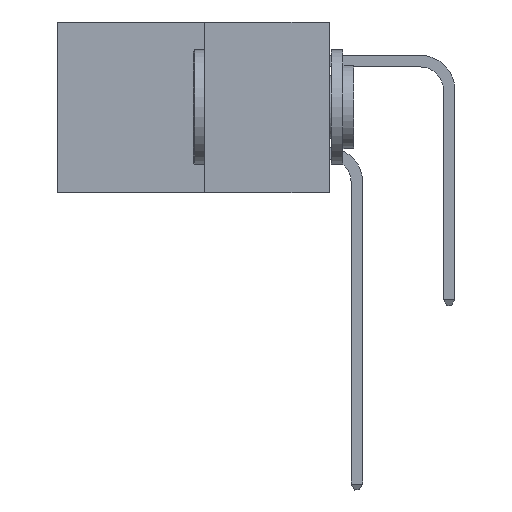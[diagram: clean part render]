
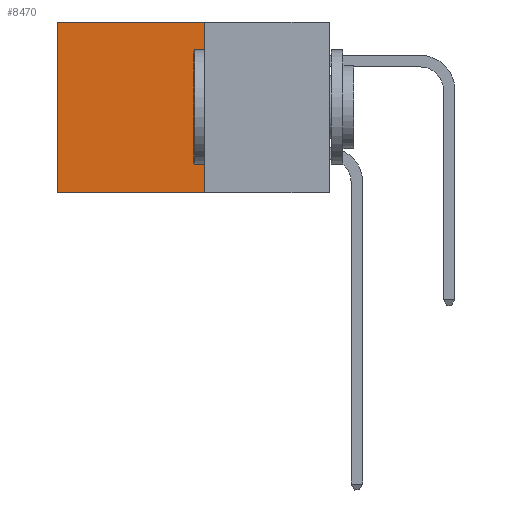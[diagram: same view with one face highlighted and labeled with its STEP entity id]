
A CAD part, left-side view. The second image highlights one B-rep face of the part: STEP entity #8470.
In plain terms, the highlighted planar face has unit normal (-1, 0, 0).
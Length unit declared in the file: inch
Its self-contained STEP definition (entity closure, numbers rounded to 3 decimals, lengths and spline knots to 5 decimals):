
#1237 = VECTOR ( 'NONE', #23311, 39.37008 ) ;
#1468 = CARTESIAN_POINT ( 'NONE',  ( 0.277, 0.59, -0.37 ) ) ;
#2689 = DIRECTION ( 'NONE',  ( 0., 1., 0. ) ) ;
#3765 = CARTESIAN_POINT ( 'NONE',  ( 0.277, 0.27, -0.37 ) ) ;
#5240 = CARTESIAN_POINT ( 'NONE',  ( 0.277, 0.27, -0.37 ) ) ;
#7362 = ORIENTED_EDGE ( 'NONE', *, *, #21702, .T. ) ;
#8470 = ADVANCED_FACE ( 'NONE', ( #24042 ), #9033, .F. ) ;
#8924 = DIRECTION ( 'NONE',  ( 0., 0., -1. ) ) ;
#9033 = PLANE ( 'NONE',  #9834 ) ;
#9094 = DIRECTION ( 'NONE',  ( 1., 0., 0. ) ) ;
#9118 = EDGE_CURVE ( 'NONE', #20205, #9613, #20356, .T. ) ;
#9613 = VERTEX_POINT ( 'NONE', #5240 ) ;
#9671 = DIRECTION ( 'NONE',  ( 0., 0., -1. ) ) ;
#9834 = AXIS2_PLACEMENT_3D ( 'NONE', #12466, #9094, #8924 ) ;
#11093 = VECTOR ( 'NONE', #9671, 39.37008 ) ;
#11422 = CARTESIAN_POINT ( 'NONE',  ( 0.277, 0.59, 0. ) ) ;
#11978 = LINE ( 'NONE', #1468, #1237 ) ;
#12466 = CARTESIAN_POINT ( 'NONE',  ( 0.277, 0.27, -0.37 ) ) ;
#12471 = VECTOR ( 'NONE', #2689, 39.37008 ) ;
#12754 = VERTEX_POINT ( 'NONE', #15803 ) ;
#13088 = LINE ( 'NONE', #22528, #12471 ) ;
#13214 = EDGE_CURVE ( 'NONE', #13866, #12754, #11978, .T. ) ;
#13242 = DIRECTION ( 'NONE',  ( 0., 1., 0. ) ) ;
#13278 = LINE ( 'NONE', #23011, #18511 ) ;
#13866 = VERTEX_POINT ( 'NONE', #11422 ) ;
#14253 = CARTESIAN_POINT ( 'NONE',  ( 0.277, 0.27, 0. ) ) ;
#15803 = CARTESIAN_POINT ( 'NONE',  ( 0.277, 0.59, -0.37 ) ) ;
#18511 = VECTOR ( 'NONE', #13242, 39.37008 ) ;
#19983 = ORIENTED_EDGE ( 'NONE', *, *, #13214, .T. ) ;
#20205 = VERTEX_POINT ( 'NONE', #14253 ) ;
#20356 = LINE ( 'NONE', #3765, #11093 ) ;
#21331 = ORIENTED_EDGE ( 'NONE', *, *, #23834, .F. ) ;
#21702 = EDGE_CURVE ( 'NONE', #20205, #13866, #13088, .T. ) ;
#22528 = CARTESIAN_POINT ( 'NONE',  ( 0.277, 0.27, 0. ) ) ;
#23011 = CARTESIAN_POINT ( 'NONE',  ( 0.277, 0.27, -0.37 ) ) ;
#23140 = ORIENTED_EDGE ( 'NONE', *, *, #9118, .F. ) ;
#23311 = DIRECTION ( 'NONE',  ( 0., 0., -1. ) ) ;
#23834 = EDGE_CURVE ( 'NONE', #9613, #12754, #13278, .T. ) ;
#24042 = FACE_OUTER_BOUND ( 'NONE', #25333, .T. ) ;
#25333 = EDGE_LOOP ( 'NONE', ( #19983, #21331, #23140, #7362 ) ) ;
